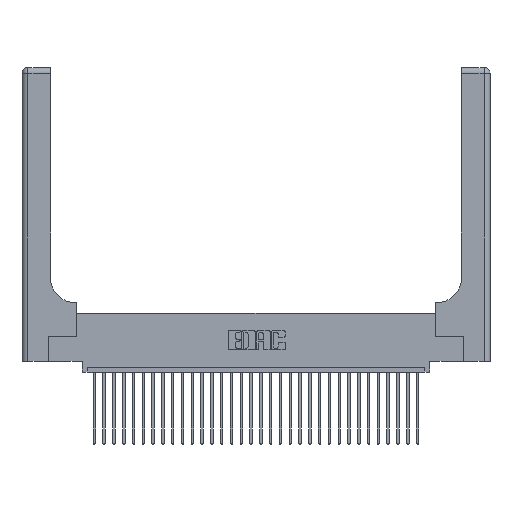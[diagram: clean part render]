
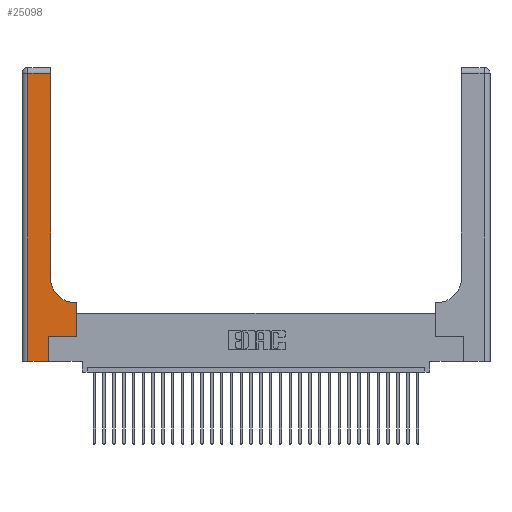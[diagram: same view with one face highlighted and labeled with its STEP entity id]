
A CAD part, top view. The second image highlights one B-rep face of the part: STEP entity #25098.
In plain terms, the highlighted planar face has unit normal (0, 0, 1).
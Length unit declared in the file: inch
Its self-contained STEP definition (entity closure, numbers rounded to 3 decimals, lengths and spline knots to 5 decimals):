
#607 = VERTEX_POINT ( 'NONE', #20054 ) ;
#696 = EDGE_CURVE ( 'NONE', #19693, #13671, #1851, .T. ) ;
#1212 = DIRECTION ( 'NONE',  ( 0., 0., -1. ) ) ;
#1381 = LINE ( 'NONE', #19296, #26877 ) ;
#1851 = LINE ( 'NONE', #23268, #8785 ) ;
#2156 = CARTESIAN_POINT ( 'NONE',  ( 0.5415, 0.6, 0.37 ) ) ;
#4519 = EDGE_CURVE ( 'NONE', #24681, #19704, #22639, .T. ) ;
#5467 = EDGE_CURVE ( 'NONE', #7855, #5851, #18697, .T. ) ;
#5851 = VERTEX_POINT ( 'NONE', #2156 ) ;
#7130 = VECTOR ( 'NONE', #10315, 39.37008 ) ;
#7855 = VERTEX_POINT ( 'NONE', #13599 ) ;
#8563 = EDGE_CURVE ( 'NONE', #24732, #19693, #29138, .T. ) ;
#8785 = VECTOR ( 'NONE', #28023, 39.37008 ) ;
#8978 = CARTESIAN_POINT ( 'NONE',  ( 0.5415, 0.85, 0.37 ) ) ;
#9557 = ORIENTED_EDGE ( 'NONE', *, *, #17285, .T. ) ;
#9627 = EDGE_LOOP ( 'NONE', ( #26248, #25227, #9557, #10215, #16713, #11700, #16313, #16912, #11989 ) ) ;
#9718 = CARTESIAN_POINT ( 'NONE',  ( 0.269, 0.25, 0.37 ) ) ;
#10215 = ORIENTED_EDGE ( 'NONE', *, *, #8563, .T. ) ;
#10315 = DIRECTION ( 'NONE',  ( 0., 1., 0. ) ) ;
#10909 = CARTESIAN_POINT ( 'NONE',  ( 0.06, 2.94, 0.37 ) ) ;
#11259 = EDGE_CURVE ( 'NONE', #13671, #30794, #1381, .T. ) ;
#11700 = ORIENTED_EDGE ( 'NONE', *, *, #11259, .T. ) ;
#11811 = EDGE_CURVE ( 'NONE', #5851, #607, #19099, .T. ) ;
#11989 = ORIENTED_EDGE ( 'NONE', *, *, #11811, .T. ) ;
#12032 = FACE_OUTER_BOUND ( 'NONE', #9627, .T. ) ;
#12156 = VECTOR ( 'NONE', #28483, 39.37008 ) ;
#12905 = CARTESIAN_POINT ( 'NONE',  ( 0.06, 3., 0.37 ) ) ;
#13469 = CARTESIAN_POINT ( 'NONE',  ( 0.2915, 0.6, 0.37 ) ) ;
#13599 = CARTESIAN_POINT ( 'NONE',  ( 0.5585, 0.6, 0.37 ) ) ;
#13615 = CARTESIAN_POINT ( 'NONE',  ( 0., 3., 0.37 ) ) ;
#13671 = VERTEX_POINT ( 'NONE', #9718 ) ;
#16313 = ORIENTED_EDGE ( 'NONE', *, *, #20872, .T. ) ;
#16671 = DIRECTION ( 'NONE',  ( 1., 0., 0. ) ) ;
#16713 = ORIENTED_EDGE ( 'NONE', *, *, #696, .T. ) ;
#16912 = ORIENTED_EDGE ( 'NONE', *, *, #5467, .T. ) ;
#17285 = EDGE_CURVE ( 'NONE', #19704, #24732, #19375, .T. ) ;
#17576 = AXIS2_PLACEMENT_3D ( 'NONE', #8978, #28205, #18711 ) ;
#18341 = VECTOR ( 'NONE', #18939, 39.37008 ) ;
#18697 = LINE ( 'NONE', #13469, #20631 ) ;
#18711 = DIRECTION ( 'NONE',  ( 1., 0., 0. ) ) ;
#18939 = DIRECTION ( 'NONE',  ( 0., 1., 0. ) ) ;
#19099 = CIRCLE ( 'NONE', #17576, 0.25 ) ;
#19221 = AXIS2_PLACEMENT_3D ( 'NONE', #13615, #1212, #28391 ) ;
#19296 = CARTESIAN_POINT ( 'NONE',  ( 0.269, 0.25, 0.37 ) ) ;
#19375 = LINE ( 'NONE', #12905, #24389 ) ;
#19693 = VERTEX_POINT ( 'NONE', #23236 ) ;
#19704 = VERTEX_POINT ( 'NONE', #10909 ) ;
#19869 = LINE ( 'NONE', #24797, #7130 ) ;
#20054 = CARTESIAN_POINT ( 'NONE',  ( 0.2915, 0.85, 0.37 ) ) ;
#20631 = VECTOR ( 'NONE', #25632, 39.37008 ) ;
#20872 = EDGE_CURVE ( 'NONE', #30794, #7855, #19869, .T. ) ;
#21194 = EDGE_CURVE ( 'NONE', #607, #24681, #22217, .T. ) ;
#22217 = LINE ( 'NONE', #31270, #18341 ) ;
#22639 = LINE ( 'NONE', #25690, #24578 ) ;
#23236 = CARTESIAN_POINT ( 'NONE',  ( 0.269, 0., 0.37 ) ) ;
#23268 = CARTESIAN_POINT ( 'NONE',  ( 0.269, 0., 0.37 ) ) ;
#23631 = CARTESIAN_POINT ( 'NONE',  ( 0., 0., 0.37 ) ) ;
#23894 = CARTESIAN_POINT ( 'NONE',  ( 0.2915, 2.94, 0.37 ) ) ;
#24112 = CARTESIAN_POINT ( 'NONE',  ( 0.06, 0., 0.37 ) ) ;
#24389 = VECTOR ( 'NONE', #30174, 39.37008 ) ;
#24578 = VECTOR ( 'NONE', #25791, 39.37008 ) ;
#24681 = VERTEX_POINT ( 'NONE', #23894 ) ;
#24732 = VERTEX_POINT ( 'NONE', #24112 ) ;
#24797 = CARTESIAN_POINT ( 'NONE',  ( 0.5585, 0.25, 0.37 ) ) ;
#25098 = ADVANCED_FACE ( 'NONE', ( #12032 ), #30789, .F. ) ;
#25227 = ORIENTED_EDGE ( 'NONE', *, *, #4519, .T. ) ;
#25632 = DIRECTION ( 'NONE',  ( -1., 0., 0. ) ) ;
#25690 = CARTESIAN_POINT ( 'NONE',  ( 0., 2.94, 0.37 ) ) ;
#25791 = DIRECTION ( 'NONE',  ( -1., 0., 0. ) ) ;
#26241 = CARTESIAN_POINT ( 'NONE',  ( 0.5585, 0.25, 0.37 ) ) ;
#26248 = ORIENTED_EDGE ( 'NONE', *, *, #21194, .T. ) ;
#26877 = VECTOR ( 'NONE', #16671, 39.37008 ) ;
#28023 = DIRECTION ( 'NONE',  ( 0., 1., 0. ) ) ;
#28205 = DIRECTION ( 'NONE',  ( 0., 0., -1. ) ) ;
#28391 = DIRECTION ( 'NONE',  ( -1., 0., 0. ) ) ;
#28483 = DIRECTION ( 'NONE',  ( 1., 0., 0. ) ) ;
#29138 = LINE ( 'NONE', #23631, #12156 ) ;
#30174 = DIRECTION ( 'NONE',  ( 0., -1., 0. ) ) ;
#30789 = PLANE ( 'NONE',  #19221 ) ;
#30794 = VERTEX_POINT ( 'NONE', #26241 ) ;
#31270 = CARTESIAN_POINT ( 'NONE',  ( 0.2915, 3., 0.37 ) ) ;
